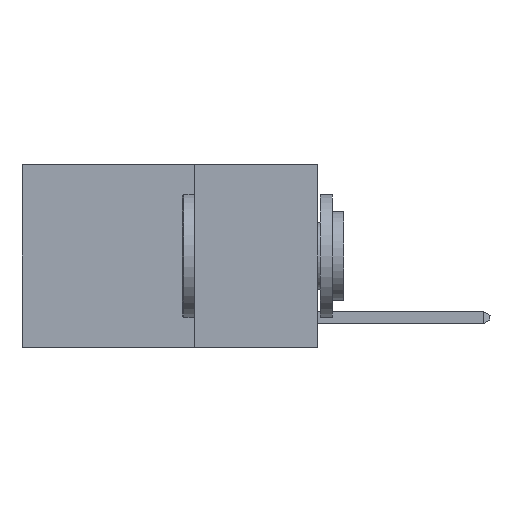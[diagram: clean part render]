
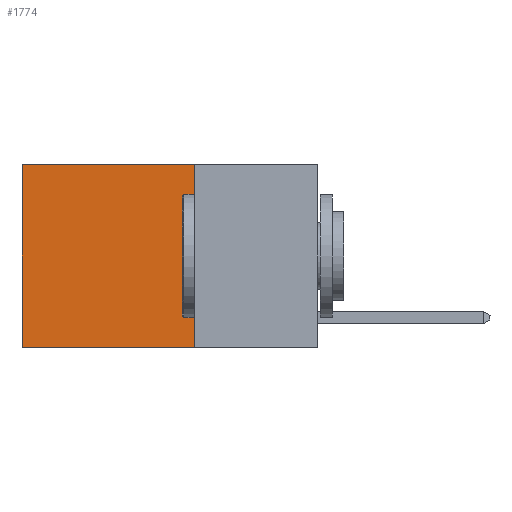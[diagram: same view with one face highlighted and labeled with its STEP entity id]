
A CAD part, left-side view. The second image highlights one B-rep face of the part: STEP entity #1774.
In plain terms, the highlighted planar face has unit normal (-1, 0, 0).
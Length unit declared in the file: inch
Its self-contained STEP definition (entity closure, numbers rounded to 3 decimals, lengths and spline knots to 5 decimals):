
#594 = VERTEX_POINT ( 'NONE', #11098 ) ;
#1774 = ADVANCED_FACE ( 'NONE', ( #2915 ), #7018, .F. ) ;
#2284 = LINE ( 'NONE', #15165, #16974 ) ;
#2422 = EDGE_CURVE ( 'NONE', #4948, #594, #2284, .T. ) ;
#2915 = FACE_OUTER_BOUND ( 'NONE', #9516, .T. ) ;
#3348 = CARTESIAN_POINT ( 'NONE',  ( 0.2625, 0.25, -0.37 ) ) ;
#4584 = CARTESIAN_POINT ( 'NONE',  ( 0.2625, 0.25, 0. ) ) ;
#4948 = VERTEX_POINT ( 'NONE', #9045 ) ;
#5784 = LINE ( 'NONE', #11282, #10648 ) ;
#6292 = CARTESIAN_POINT ( 'NONE',  ( 0.2625, 0.25, -0.37 ) ) ;
#7018 = PLANE ( 'NONE',  #10903 ) ;
#7563 = DIRECTION ( 'NONE',  ( 0., 0., -1. ) ) ;
#8317 = DIRECTION ( 'NONE',  ( 0., 1., 0. ) ) ;
#8512 = CARTESIAN_POINT ( 'NONE',  ( 0.2625, 0.25, 0. ) ) ;
#9045 = CARTESIAN_POINT ( 'NONE',  ( 0.2625, 0.6, 0. ) ) ;
#9516 = EDGE_LOOP ( 'NONE', ( #15662, #11653, #11437, #15342 ) ) ;
#10648 = VECTOR ( 'NONE', #8317, 39.37008 ) ;
#10720 = EDGE_CURVE ( 'NONE', #13022, #594, #13056, .T. ) ;
#10903 = AXIS2_PLACEMENT_3D ( 'NONE', #8512, #11292, #18391 ) ;
#11098 = CARTESIAN_POINT ( 'NONE',  ( 0.2625, 0.6, -0.37 ) ) ;
#11282 = CARTESIAN_POINT ( 'NONE',  ( 0.2625, 0.25, 0. ) ) ;
#11292 = DIRECTION ( 'NONE',  ( 1., 0., 0. ) ) ;
#11437 = ORIENTED_EDGE ( 'NONE', *, *, #17547, .F. ) ;
#11653 = ORIENTED_EDGE ( 'NONE', *, *, #10720, .F. ) ;
#12649 = VECTOR ( 'NONE', #13232, 39.37008 ) ;
#13022 = VERTEX_POINT ( 'NONE', #6292 ) ;
#13056 = LINE ( 'NONE', #3348, #12649 ) ;
#13232 = DIRECTION ( 'NONE',  ( 0., 1., 0. ) ) ;
#13372 = VECTOR ( 'NONE', #7563, 39.37008 ) ;
#15165 = CARTESIAN_POINT ( 'NONE',  ( 0.2625, 0.6, 0. ) ) ;
#15254 = DIRECTION ( 'NONE',  ( 0., 0., -1. ) ) ;
#15342 = ORIENTED_EDGE ( 'NONE', *, *, #15992, .T. ) ;
#15662 = ORIENTED_EDGE ( 'NONE', *, *, #2422, .T. ) ;
#15992 = EDGE_CURVE ( 'NONE', #17696, #4948, #5784, .T. ) ;
#16052 = LINE ( 'NONE', #4584, #13372 ) ;
#16974 = VECTOR ( 'NONE', #15254, 39.37008 ) ;
#17547 = EDGE_CURVE ( 'NONE', #17696, #13022, #16052, .T. ) ;
#17696 = VERTEX_POINT ( 'NONE', #17712 ) ;
#17712 = CARTESIAN_POINT ( 'NONE',  ( 0.2625, 0.25, 0. ) ) ;
#18391 = DIRECTION ( 'NONE',  ( 0., 0., -1. ) ) ;
